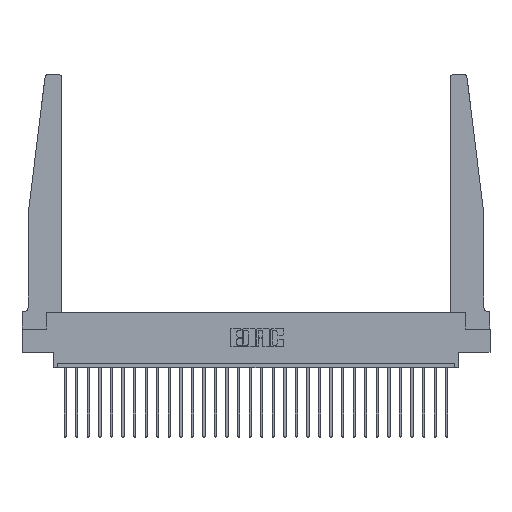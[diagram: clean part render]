
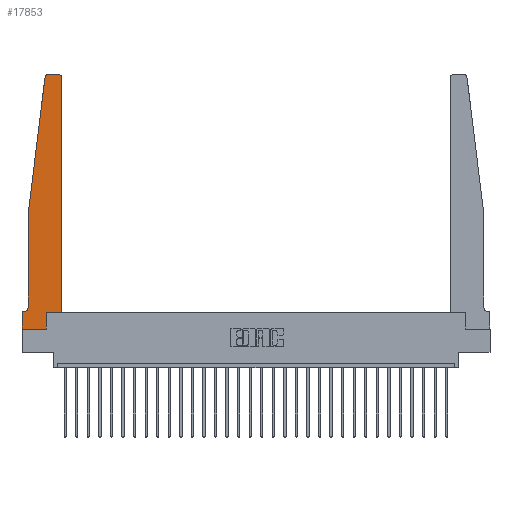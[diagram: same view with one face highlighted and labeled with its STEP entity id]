
A CAD part, top view. The second image highlights one B-rep face of the part: STEP entity #17853.
In plain terms, the highlighted planar face has unit normal (0, 0, 1).
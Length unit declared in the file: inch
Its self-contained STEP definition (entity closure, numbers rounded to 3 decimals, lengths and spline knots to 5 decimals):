
#277 = CARTESIAN_POINT ( 'NONE',  ( 0.2605, 0., 0.37 ) ) ;
#657 = CARTESIAN_POINT ( 'NONE',  ( 0., 0., 0.37 ) ) ;
#730 = DIRECTION ( 'NONE',  ( 1., 0., 0. ) ) ;
#765 = ORIENTED_EDGE ( 'NONE', *, *, #20935, .T. ) ;
#844 = CARTESIAN_POINT ( 'NONE',  ( 0.065, 1.25, 0.37 ) ) ;
#1534 = CARTESIAN_POINT ( 'NONE',  ( 0.2605, 0.18, 0.37 ) ) ;
#1755 = DIRECTION ( 'NONE',  ( 1., 0., 0. ) ) ;
#1847 = LINE ( 'NONE', #10350, #7663 ) ;
#1937 = VECTOR ( 'NONE', #14260, 39.37008 ) ;
#1950 = VERTEX_POINT ( 'NONE', #277 ) ;
#2080 = CARTESIAN_POINT ( 'NONE',  ( 0., 0., 0.37 ) ) ;
#2672 = EDGE_CURVE ( 'NONE', #13446, #6009, #21580, .T. ) ;
#2909 = VECTOR ( 'NONE', #25987, 39.37008 ) ;
#3375 = DIRECTION ( 'NONE',  ( -1., 0., 0. ) ) ;
#3572 = ORIENTED_EDGE ( 'NONE', *, *, #6509, .T. ) ;
#3581 = DIRECTION ( 'NONE',  ( -0.122, -0.992, 0. ) ) ;
#3623 = DIRECTION ( 'NONE',  ( 0., 1., 0. ) ) ;
#3865 = AXIS2_PLACEMENT_3D ( 'NONE', #21240, #18895, #1755 ) ;
#4020 = VECTOR ( 'NONE', #15093, 39.37008 ) ;
#4441 = ORIENTED_EDGE ( 'NONE', *, *, #20719, .T. ) ;
#5816 = DIRECTION ( 'NONE',  ( 0., 0., 1. ) ) ;
#5951 = CARTESIAN_POINT ( 'NONE',  ( 0.065, 1.25, 0.37 ) ) ;
#6009 = VERTEX_POINT ( 'NONE', #6909 ) ;
#6071 = AXIS2_PLACEMENT_3D ( 'NONE', #14608, #10827, #25584 ) ;
#6362 = VERTEX_POINT ( 'NONE', #11723 ) ;
#6509 = EDGE_CURVE ( 'NONE', #23673, #20089, #11437, .T. ) ;
#6865 = CARTESIAN_POINT ( 'NONE',  ( 0.395, 2.72, 0.37 ) ) ;
#6909 = CARTESIAN_POINT ( 'NONE',  ( 0.24675, 2.72367, 0.37 ) ) ;
#6919 = AXIS2_PLACEMENT_3D ( 'NONE', #7625, #5816, #20584 ) ;
#7231 = EDGE_CURVE ( 'NONE', #21614, #13446, #21665, .T. ) ;
#7389 = CIRCLE ( 'NONE', #6071, 0.05 ) ;
#7416 = LINE ( 'NONE', #22319, #23555 ) ;
#7625 = CARTESIAN_POINT ( 'NONE',  ( 0.27653, 2.72, 0.37 ) ) ;
#7663 = VECTOR ( 'NONE', #18848, 39.37008 ) ;
#7768 = LINE ( 'NONE', #5951, #10668 ) ;
#8383 = EDGE_CURVE ( 'NONE', #20089, #6362, #7389, .T. ) ;
#9346 = DIRECTION ( 'NONE',  ( 0., -1., 0. ) ) ;
#9420 = CARTESIAN_POINT ( 'NONE',  ( 0.25, 2.75, 0.37 ) ) ;
#9805 = EDGE_CURVE ( 'NONE', #1950, #23020, #22703, .T. ) ;
#10350 = CARTESIAN_POINT ( 'NONE',  ( 0.425, 0.18, 0.37 ) ) ;
#10668 = VECTOR ( 'NONE', #3581, 39.37008 ) ;
#10822 = CARTESIAN_POINT ( 'NONE',  ( 0.065, 1.25, 0.37 ) ) ;
#10827 = DIRECTION ( 'NONE',  ( 0., 0., -1. ) ) ;
#11437 = LINE ( 'NONE', #844, #22523 ) ;
#11723 = CARTESIAN_POINT ( 'NONE',  ( 0.015, 0.1875, 0.37 ) ) ;
#11754 = LINE ( 'NONE', #20250, #1937 ) ;
#12295 = CARTESIAN_POINT ( 'NONE',  ( 0.425, 0.18, 0.37 ) ) ;
#12756 = ORIENTED_EDGE ( 'NONE', *, *, #21172, .T. ) ;
#13446 = VERTEX_POINT ( 'NONE', #16393 ) ;
#14260 = DIRECTION ( 'NONE',  ( 0., 1., 0. ) ) ;
#14363 = LINE ( 'NONE', #2080, #25356 ) ;
#14608 = CARTESIAN_POINT ( 'NONE',  ( 0.015, 0.2375, 0.37 ) ) ;
#14691 = ORIENTED_EDGE ( 'NONE', *, *, #20900, .T. ) ;
#15093 = DIRECTION ( 'NONE',  ( 0., -1., 0. ) ) ;
#15363 = DIRECTION ( 'NONE',  ( 0., 0., 1. ) ) ;
#15382 = EDGE_LOOP ( 'NONE', ( #23103, #26803, #4441, #3572, #16467, #765, #12756, #24755, #27314, #18081, #23289, #14691 ) ) ;
#16393 = CARTESIAN_POINT ( 'NONE',  ( 0.27653, 2.75, 0.37 ) ) ;
#16460 = VERTEX_POINT ( 'NONE', #18776 ) ;
#16467 = ORIENTED_EDGE ( 'NONE', *, *, #8383, .T. ) ;
#16909 = AXIS2_PLACEMENT_3D ( 'NONE', #6865, #15363, #730 ) ;
#17595 = CARTESIAN_POINT ( 'NONE',  ( 0., 0., 0.37 ) ) ;
#17853 = ADVANCED_FACE ( 'NONE', ( #19166 ), #27383, .T. ) ;
#17950 = CARTESIAN_POINT ( 'NONE',  ( 0.425, 2.72, 0.37 ) ) ;
#18081 = ORIENTED_EDGE ( 'NONE', *, *, #25367, .T. ) ;
#18776 = CARTESIAN_POINT ( 'NONE',  ( 0., 0.1875, 0.37 ) ) ;
#18848 = DIRECTION ( 'NONE',  ( 1., 0., 0. ) ) ;
#18895 = DIRECTION ( 'NONE',  ( 0., 0., 1. ) ) ;
#19040 = VECTOR ( 'NONE', #3623, 39.37008 ) ;
#19166 = FACE_OUTER_BOUND ( 'NONE', #15382, .T. ) ;
#20089 = VERTEX_POINT ( 'NONE', #23401 ) ;
#20250 = CARTESIAN_POINT ( 'NONE',  ( 0.425, 0.18, 0.37 ) ) ;
#20584 = DIRECTION ( 'NONE',  ( 1., 0., 0. ) ) ;
#20710 = VERTEX_POINT ( 'NONE', #657 ) ;
#20719 = EDGE_CURVE ( 'NONE', #6009, #23673, #7768, .T. ) ;
#20893 = CARTESIAN_POINT ( 'NONE',  ( 0.2605, 0.18, 0.37 ) ) ;
#20900 = EDGE_CURVE ( 'NONE', #24567, #21614, #22227, .T. ) ;
#20935 = EDGE_CURVE ( 'NONE', #6362, #16460, #7416, .T. ) ;
#21172 = EDGE_CURVE ( 'NONE', #16460, #20710, #23852, .T. ) ;
#21240 = CARTESIAN_POINT ( 'NONE',  ( 0., 0.1875, 0.37 ) ) ;
#21580 = CIRCLE ( 'NONE', #6919, 0.03 ) ;
#21614 = VERTEX_POINT ( 'NONE', #21732 ) ;
#21665 = LINE ( 'NONE', #9420, #2909 ) ;
#21732 = CARTESIAN_POINT ( 'NONE',  ( 0.395, 2.75, 0.37 ) ) ;
#22227 = CIRCLE ( 'NONE', #16909, 0.03 ) ;
#22319 = CARTESIAN_POINT ( 'NONE',  ( 0.065, 0.1875, 0.37 ) ) ;
#22523 = VECTOR ( 'NONE', #9346, 39.37008 ) ;
#22703 = LINE ( 'NONE', #1534, #19040 ) ;
#23020 = VERTEX_POINT ( 'NONE', #20893 ) ;
#23025 = EDGE_CURVE ( 'NONE', #20710, #1950, #14363, .T. ) ;
#23103 = ORIENTED_EDGE ( 'NONE', *, *, #7231, .T. ) ;
#23289 = ORIENTED_EDGE ( 'NONE', *, *, #26451, .T. ) ;
#23401 = CARTESIAN_POINT ( 'NONE',  ( 0.065, 0.2375, 0.37 ) ) ;
#23555 = VECTOR ( 'NONE', #3375, 39.37008 ) ;
#23673 = VERTEX_POINT ( 'NONE', #10822 ) ;
#23852 = LINE ( 'NONE', #17595, #4020 ) ;
#24567 = VERTEX_POINT ( 'NONE', #17950 ) ;
#24755 = ORIENTED_EDGE ( 'NONE', *, *, #23025, .T. ) ;
#25322 = VERTEX_POINT ( 'NONE', #12295 ) ;
#25343 = DIRECTION ( 'NONE',  ( 1., 0., 0. ) ) ;
#25356 = VECTOR ( 'NONE', #25343, 39.37008 ) ;
#25367 = EDGE_CURVE ( 'NONE', #23020, #25322, #1847, .T. ) ;
#25584 = DIRECTION ( 'NONE',  ( -1., 0., 0. ) ) ;
#25987 = DIRECTION ( 'NONE',  ( -1., 0., 0. ) ) ;
#26451 = EDGE_CURVE ( 'NONE', #25322, #24567, #11754, .T. ) ;
#26803 = ORIENTED_EDGE ( 'NONE', *, *, #2672, .T. ) ;
#27314 = ORIENTED_EDGE ( 'NONE', *, *, #9805, .T. ) ;
#27383 = PLANE ( 'NONE',  #3865 ) ;
